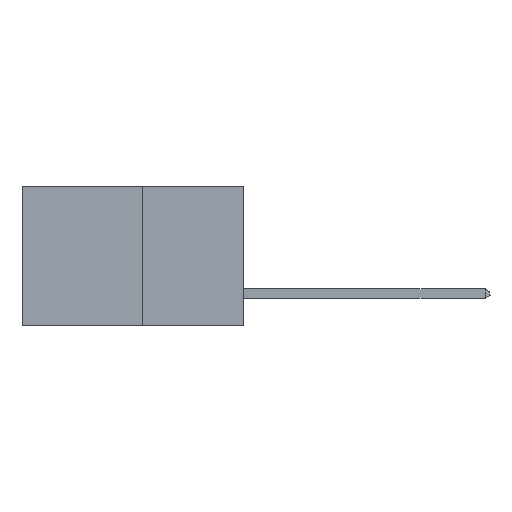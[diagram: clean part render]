
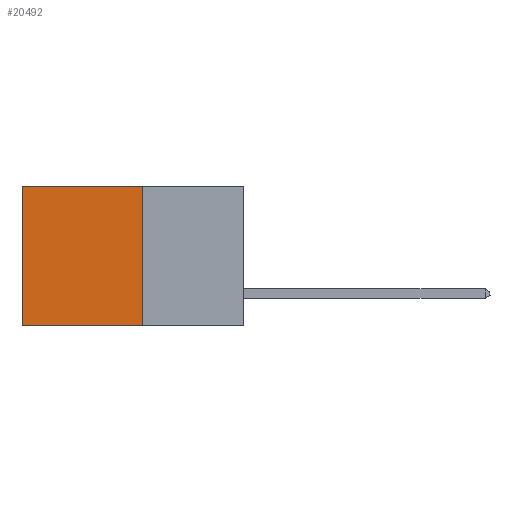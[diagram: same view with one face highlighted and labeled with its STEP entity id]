
A CAD part, left-side view. The second image highlights one B-rep face of the part: STEP entity #20492.
In plain terms, the highlighted planar face has unit normal (-1, 0, 0).
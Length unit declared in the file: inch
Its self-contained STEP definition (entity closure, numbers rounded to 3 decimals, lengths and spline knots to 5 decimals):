
#565 = CARTESIAN_POINT ( 'NONE',  ( 0.277, 0.27, -0.37 ) ) ;
#5392 = VECTOR ( 'NONE', #26432, 39.37008 ) ;
#7564 = CARTESIAN_POINT ( 'NONE',  ( 0.277, 0.27, -0.37 ) ) ;
#7793 = CARTESIAN_POINT ( 'NONE',  ( 0.277, 0.27, -0.37 ) ) ;
#8474 = LINE ( 'NONE', #23328, #26313 ) ;
#8779 = FACE_OUTER_BOUND ( 'NONE', #27347, .T. ) ;
#9946 = DIRECTION ( 'NONE',  ( 0., 0., -1. ) ) ;
#10631 = CARTESIAN_POINT ( 'NONE',  ( 0.277, 0.59, -0.37 ) ) ;
#11251 = VECTOR ( 'NONE', #27228, 39.37008 ) ;
#12810 = CARTESIAN_POINT ( 'NONE',  ( 0.277, 0.59, -0.37 ) ) ;
#13010 = DIRECTION ( 'NONE',  ( 0., 0., -1. ) ) ;
#13515 = EDGE_CURVE ( 'NONE', #20453, #14015, #8474, .T. ) ;
#13881 = ORIENTED_EDGE ( 'NONE', *, *, #22952, .F. ) ;
#14015 = VERTEX_POINT ( 'NONE', #27265 ) ;
#14881 = ORIENTED_EDGE ( 'NONE', *, *, #22733, .F. ) ;
#14934 = LINE ( 'NONE', #10631, #26436 ) ;
#15079 = VERTEX_POINT ( 'NONE', #565 ) ;
#17281 = VERTEX_POINT ( 'NONE', #12810 ) ;
#17310 = EDGE_CURVE ( 'NONE', #14015, #17281, #14934, .T. ) ;
#17575 = LINE ( 'NONE', #22668, #11251 ) ;
#20453 = VERTEX_POINT ( 'NONE', #21421 ) ;
#20492 = ADVANCED_FACE ( 'NONE', ( #8779 ), #23845, .F. ) ;
#21421 = CARTESIAN_POINT ( 'NONE',  ( 0.277, 0.27, 0. ) ) ;
#22497 = AXIS2_PLACEMENT_3D ( 'NONE', #7564, #23943, #9946 ) ;
#22668 = CARTESIAN_POINT ( 'NONE',  ( 0.277, 0.27, -0.37 ) ) ;
#22733 = EDGE_CURVE ( 'NONE', #15079, #17281, #30048, .T. ) ;
#22952 = EDGE_CURVE ( 'NONE', #20453, #15079, #17575, .T. ) ;
#23328 = CARTESIAN_POINT ( 'NONE',  ( 0.277, 0.27, 0. ) ) ;
#23735 = ORIENTED_EDGE ( 'NONE', *, *, #13515, .T. ) ;
#23845 = PLANE ( 'NONE',  #22497 ) ;
#23943 = DIRECTION ( 'NONE',  ( 1., 0., 0. ) ) ;
#25836 = ORIENTED_EDGE ( 'NONE', *, *, #17310, .T. ) ;
#26313 = VECTOR ( 'NONE', #27774, 39.37008 ) ;
#26432 = DIRECTION ( 'NONE',  ( 0., 1., 0. ) ) ;
#26436 = VECTOR ( 'NONE', #13010, 39.37008 ) ;
#27228 = DIRECTION ( 'NONE',  ( 0., 0., -1. ) ) ;
#27265 = CARTESIAN_POINT ( 'NONE',  ( 0.277, 0.59, 0. ) ) ;
#27347 = EDGE_LOOP ( 'NONE', ( #25836, #14881, #13881, #23735 ) ) ;
#27774 = DIRECTION ( 'NONE',  ( 0., 1., 0. ) ) ;
#30048 = LINE ( 'NONE', #7793, #5392 ) ;
